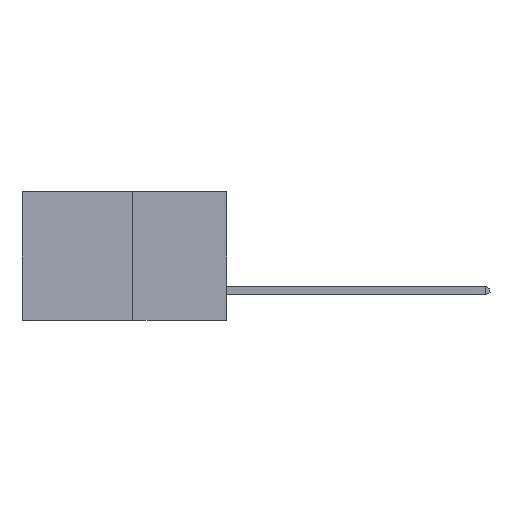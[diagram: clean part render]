
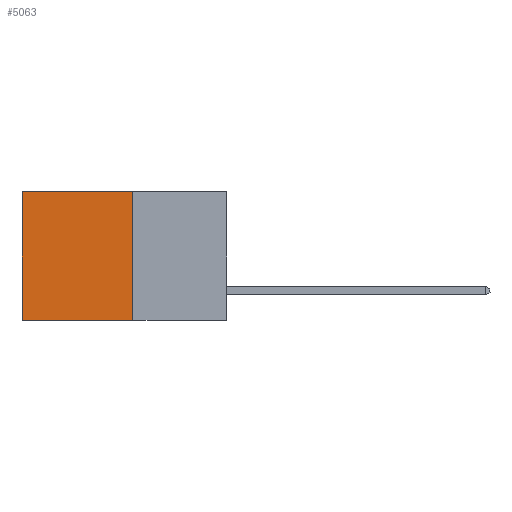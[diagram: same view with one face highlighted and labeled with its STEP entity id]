
A CAD part, left-side view. The second image highlights one B-rep face of the part: STEP entity #5063.
In plain terms, the highlighted planar face has unit normal (-1, 0, 0).
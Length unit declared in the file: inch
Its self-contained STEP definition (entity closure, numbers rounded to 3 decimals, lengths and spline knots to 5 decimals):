
#132 = VECTOR ( 'NONE', #6010, 39.37008 ) ;
#317 = ORIENTED_EDGE ( 'NONE', *, *, #5769, .F. ) ;
#331 = DIRECTION ( 'NONE',  ( 0., 0., -1. ) ) ;
#853 = DIRECTION ( 'NONE',  ( 0., 0., -1. ) ) ;
#904 = CARTESIAN_POINT ( 'NONE',  ( 0.277, 0.27, -0.37 ) ) ;
#956 = ORIENTED_EDGE ( 'NONE', *, *, #2951, .F. ) ;
#1284 = EDGE_LOOP ( 'NONE', ( #3215, #317, #956, #5923 ) ) ;
#1954 = DIRECTION ( 'NONE',  ( 0., 0., -1. ) ) ;
#2076 = EDGE_CURVE ( 'NONE', #8940, #5255, #9808, .T. ) ;
#2492 = LINE ( 'NONE', #5096, #132 ) ;
#2781 = CARTESIAN_POINT ( 'NONE',  ( 0.277, 0.59, 0. ) ) ;
#2951 = EDGE_CURVE ( 'NONE', #7881, #3616, #7628, .T. ) ;
#3215 = ORIENTED_EDGE ( 'NONE', *, *, #2076, .T. ) ;
#3311 = AXIS2_PLACEMENT_3D ( 'NONE', #8056, #8033, #853 ) ;
#3616 = VERTEX_POINT ( 'NONE', #3856 ) ;
#3856 = CARTESIAN_POINT ( 'NONE',  ( 0.277, 0.27, -0.37 ) ) ;
#4206 = CARTESIAN_POINT ( 'NONE',  ( 0.277, 0.59, -0.37 ) ) ;
#5063 = ADVANCED_FACE ( 'NONE', ( #6043 ), #9799, .F. ) ;
#5096 = CARTESIAN_POINT ( 'NONE',  ( 0.277, 0.27, 0. ) ) ;
#5255 = VERTEX_POINT ( 'NONE', #4206 ) ;
#5647 = LINE ( 'NONE', #6572, #7917 ) ;
#5693 = VECTOR ( 'NONE', #331, 39.37008 ) ;
#5769 = EDGE_CURVE ( 'NONE', #3616, #5255, #5647, .T. ) ;
#5923 = ORIENTED_EDGE ( 'NONE', *, *, #6697, .T. ) ;
#6010 = DIRECTION ( 'NONE',  ( 0., 1., 0. ) ) ;
#6043 = FACE_OUTER_BOUND ( 'NONE', #1284, .T. ) ;
#6285 = CARTESIAN_POINT ( 'NONE',  ( 0.277, 0.59, -0.37 ) ) ;
#6572 = CARTESIAN_POINT ( 'NONE',  ( 0.277, 0.27, -0.37 ) ) ;
#6573 = DIRECTION ( 'NONE',  ( 0., 1., 0. ) ) ;
#6697 = EDGE_CURVE ( 'NONE', #7881, #8940, #2492, .T. ) ;
#7628 = LINE ( 'NONE', #904, #7858 ) ;
#7858 = VECTOR ( 'NONE', #1954, 39.37008 ) ;
#7881 = VERTEX_POINT ( 'NONE', #8672 ) ;
#7917 = VECTOR ( 'NONE', #6573, 39.37008 ) ;
#8033 = DIRECTION ( 'NONE',  ( 1., 0., 0. ) ) ;
#8056 = CARTESIAN_POINT ( 'NONE',  ( 0.277, 0.27, -0.37 ) ) ;
#8672 = CARTESIAN_POINT ( 'NONE',  ( 0.277, 0.27, 0. ) ) ;
#8940 = VERTEX_POINT ( 'NONE', #2781 ) ;
#9799 = PLANE ( 'NONE',  #3311 ) ;
#9808 = LINE ( 'NONE', #6285, #5693 ) ;
